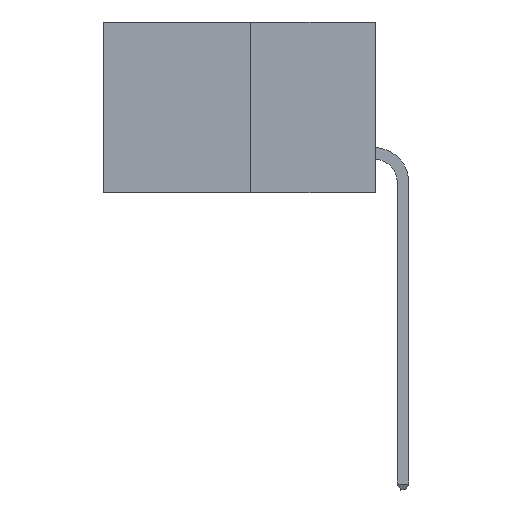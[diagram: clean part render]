
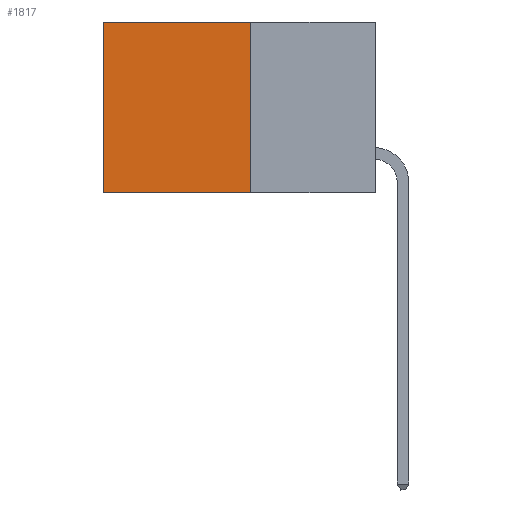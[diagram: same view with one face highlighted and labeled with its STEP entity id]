
A CAD part, left-side view. The second image highlights one B-rep face of the part: STEP entity #1817.
In plain terms, the highlighted planar face has unit normal (-1, 0, 0).
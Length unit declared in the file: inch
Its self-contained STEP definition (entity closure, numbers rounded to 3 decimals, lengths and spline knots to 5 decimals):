
#310 = VERTEX_POINT ( 'NONE', #2263 ) ;
#412 = DIRECTION ( 'NONE',  ( 0., 0., -1. ) ) ;
#650 = AXIS2_PLACEMENT_3D ( 'NONE', #2220, #8917, #8640 ) ;
#867 = ORIENTED_EDGE ( 'NONE', *, *, #1578, .F. ) ;
#1414 = ORIENTED_EDGE ( 'NONE', *, *, #5999, .T. ) ;
#1578 = EDGE_CURVE ( 'NONE', #9298, #6433, #10606, .T. ) ;
#1817 = ADVANCED_FACE ( 'NONE', ( #2026 ), #4560, .F. ) ;
#2026 = FACE_OUTER_BOUND ( 'NONE', #10143, .T. ) ;
#2220 = CARTESIAN_POINT ( 'NONE',  ( 0.277, 0.27, -0.37 ) ) ;
#2263 = CARTESIAN_POINT ( 'NONE',  ( 0.277, 0.59, -0.37 ) ) ;
#2743 = CARTESIAN_POINT ( 'NONE',  ( 0.277, 0.27, -0.37 ) ) ;
#2994 = CARTESIAN_POINT ( 'NONE',  ( 0.277, 0.59, 0. ) ) ;
#3259 = CARTESIAN_POINT ( 'NONE',  ( 0.277, 0.27, 0. ) ) ;
#3508 = VECTOR ( 'NONE', #10401, 39.37008 ) ;
#4028 = VECTOR ( 'NONE', #412, 39.37008 ) ;
#4560 = PLANE ( 'NONE',  #650 ) ;
#4935 = VECTOR ( 'NONE', #10298, 39.37008 ) ;
#5497 = LINE ( 'NONE', #10359, #4935 ) ;
#5999 = EDGE_CURVE ( 'NONE', #6938, #310, #7576, .T. ) ;
#6017 = CARTESIAN_POINT ( 'NONE',  ( 0.277, 0.27, -0.37 ) ) ;
#6322 = EDGE_CURVE ( 'NONE', #9298, #6938, #11304, .T. ) ;
#6433 = VERTEX_POINT ( 'NONE', #6017 ) ;
#6884 = VECTOR ( 'NONE', #7025, 39.37008 ) ;
#6938 = VERTEX_POINT ( 'NONE', #2994 ) ;
#7025 = DIRECTION ( 'NONE',  ( 0., 1., 0. ) ) ;
#7105 = ORIENTED_EDGE ( 'NONE', *, *, #6322, .T. ) ;
#7239 = CARTESIAN_POINT ( 'NONE',  ( 0.277, 0.27, 0. ) ) ;
#7576 = LINE ( 'NONE', #10516, #3508 ) ;
#8044 = EDGE_CURVE ( 'NONE', #6433, #310, #5497, .T. ) ;
#8640 = DIRECTION ( 'NONE',  ( 0., 0., -1. ) ) ;
#8917 = DIRECTION ( 'NONE',  ( 1., 0., 0. ) ) ;
#9298 = VERTEX_POINT ( 'NONE', #3259 ) ;
#10143 = EDGE_LOOP ( 'NONE', ( #1414, #11091, #867, #7105 ) ) ;
#10298 = DIRECTION ( 'NONE',  ( 0., 1., 0. ) ) ;
#10359 = CARTESIAN_POINT ( 'NONE',  ( 0.277, 0.27, -0.37 ) ) ;
#10401 = DIRECTION ( 'NONE',  ( 0., 0., -1. ) ) ;
#10516 = CARTESIAN_POINT ( 'NONE',  ( 0.277, 0.59, -0.37 ) ) ;
#10606 = LINE ( 'NONE', #2743, #4028 ) ;
#11091 = ORIENTED_EDGE ( 'NONE', *, *, #8044, .F. ) ;
#11304 = LINE ( 'NONE', #7239, #6884 ) ;
